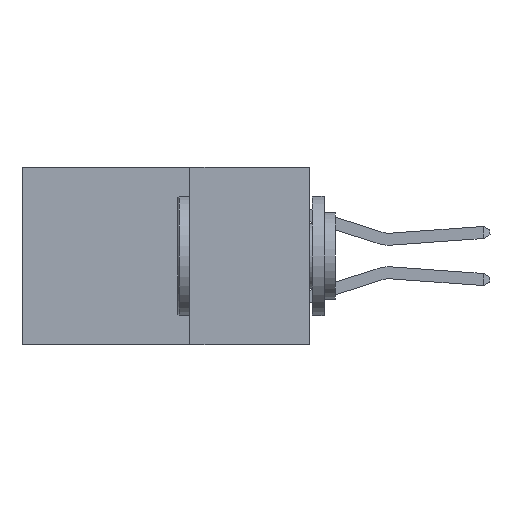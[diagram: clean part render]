
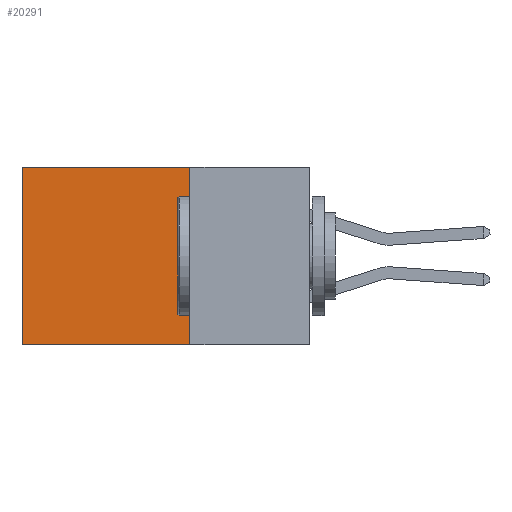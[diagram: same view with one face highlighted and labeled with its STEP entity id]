
A CAD part, left-side view. The second image highlights one B-rep face of the part: STEP entity #20291.
In plain terms, the highlighted planar face has unit normal (-1, 0, 0).
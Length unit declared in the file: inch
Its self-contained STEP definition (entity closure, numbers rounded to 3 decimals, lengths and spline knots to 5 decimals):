
#311 = CARTESIAN_POINT ( 'NONE',  ( 0.298, 0.25, 0. ) ) ;
#2100 = DIRECTION ( 'NONE',  ( 0., 1., 0. ) ) ;
#2221 = VERTEX_POINT ( 'NONE', #20493 ) ;
#2271 = EDGE_LOOP ( 'NONE', ( #17338, #6988, #10991, #13673 ) ) ;
#2274 = CARTESIAN_POINT ( 'NONE',  ( 0.298, 0.6, 0. ) ) ;
#2449 = VECTOR ( 'NONE', #15645, 39.37008 ) ;
#2568 = VERTEX_POINT ( 'NONE', #16921 ) ;
#2901 = EDGE_CURVE ( 'NONE', #2568, #3125, #16934, .T. ) ;
#2926 = EDGE_CURVE ( 'NONE', #17495, #2221, #16383, .T. ) ;
#3125 = VERTEX_POINT ( 'NONE', #4927 ) ;
#3256 = AXIS2_PLACEMENT_3D ( 'NONE', #17214, #7044, #18902 ) ;
#3468 = PLANE ( 'NONE',  #3256 ) ;
#3587 = FACE_OUTER_BOUND ( 'NONE', #2271, .T. ) ;
#3768 = VECTOR ( 'NONE', #19366, 39.37008 ) ;
#3847 = VECTOR ( 'NONE', #2100, 39.37008 ) ;
#3949 = CARTESIAN_POINT ( 'NONE',  ( 0.298, 0.25, 0. ) ) ;
#4927 = CARTESIAN_POINT ( 'NONE',  ( 0.298, 0.6, -0.37 ) ) ;
#6988 = ORIENTED_EDGE ( 'NONE', *, *, #20378, .F. ) ;
#7044 = DIRECTION ( 'NONE',  ( 1., 0., 0. ) ) ;
#8418 = CARTESIAN_POINT ( 'NONE',  ( 0.298, 0.25, 0. ) ) ;
#10991 = ORIENTED_EDGE ( 'NONE', *, *, #2926, .F. ) ;
#11928 = VECTOR ( 'NONE', #19319, 39.37008 ) ;
#13673 = ORIENTED_EDGE ( 'NONE', *, *, #21227, .T. ) ;
#15645 = DIRECTION ( 'NONE',  ( 0., 1., 0. ) ) ;
#16383 = LINE ( 'NONE', #8418, #11928 ) ;
#16921 = CARTESIAN_POINT ( 'NONE',  ( 0.298, 0.6, 0. ) ) ;
#16934 = LINE ( 'NONE', #2274, #3768 ) ;
#17018 = LINE ( 'NONE', #311, #3847 ) ;
#17214 = CARTESIAN_POINT ( 'NONE',  ( 0.298, 0.25, 0. ) ) ;
#17338 = ORIENTED_EDGE ( 'NONE', *, *, #2901, .T. ) ;
#17495 = VERTEX_POINT ( 'NONE', #3949 ) ;
#18902 = DIRECTION ( 'NONE',  ( 0., 0., -1. ) ) ;
#19041 = CARTESIAN_POINT ( 'NONE',  ( 0.298, 0.25, -0.37 ) ) ;
#19319 = DIRECTION ( 'NONE',  ( 0., 0., -1. ) ) ;
#19366 = DIRECTION ( 'NONE',  ( 0., 0., -1. ) ) ;
#20212 = LINE ( 'NONE', #19041, #2449 ) ;
#20291 = ADVANCED_FACE ( 'NONE', ( #3587 ), #3468, .F. ) ;
#20378 = EDGE_CURVE ( 'NONE', #2221, #3125, #20212, .T. ) ;
#20493 = CARTESIAN_POINT ( 'NONE',  ( 0.298, 0.25, -0.37 ) ) ;
#21227 = EDGE_CURVE ( 'NONE', #17495, #2568, #17018, .T. ) ;
